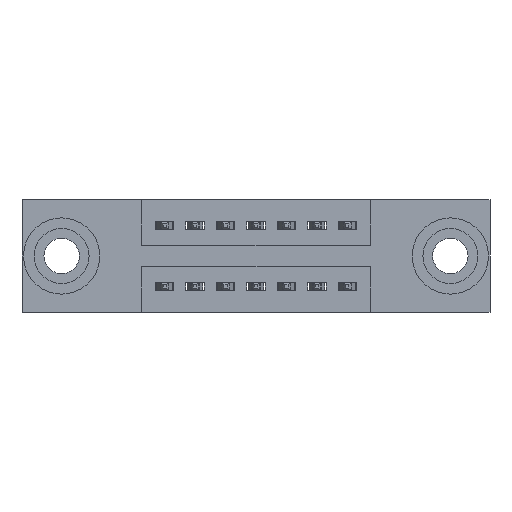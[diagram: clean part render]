
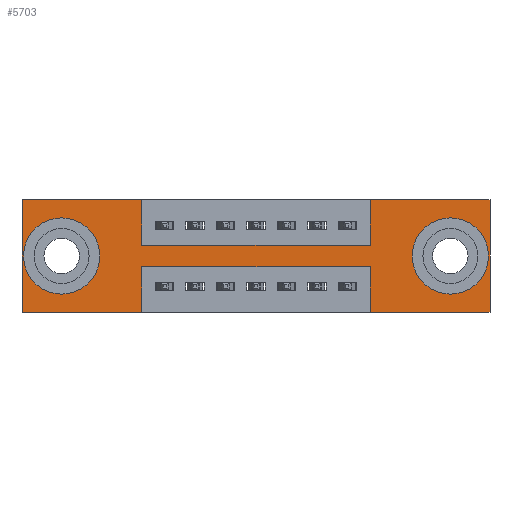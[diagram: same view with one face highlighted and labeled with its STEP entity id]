
A CAD part, front view. The second image highlights one B-rep face of the part: STEP entity #5703.
In plain terms, the highlighted planar face has unit normal (0, -1, 0).
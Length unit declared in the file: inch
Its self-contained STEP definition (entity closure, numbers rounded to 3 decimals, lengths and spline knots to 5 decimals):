
#3 = CARTESIAN_POINT ( 'NONE',  ( 0., 0., 0. ) ) ;
#21 = CARTESIAN_POINT ( 'NONE',  ( 1.405, 0., -0.185 ) ) ;
#59 = DIRECTION ( 'NONE',  ( 0., 0., -1. ) ) ;
#138 = LINE ( 'NONE', #5798, #3147 ) ;
#299 = EDGE_CURVE ( 'NONE', #4560, #1194, #5569, .T. ) ;
#536 = VECTOR ( 'NONE', #2727, 39.37008 ) ;
#591 = VECTOR ( 'NONE', #1917, 39.37008 ) ;
#703 = ORIENTED_EDGE ( 'NONE', *, *, #299, .F. ) ;
#714 = AXIS2_PLACEMENT_3D ( 'NONE', #5521, #6251, #9649 ) ;
#724 = VERTEX_POINT ( 'NONE', #5228 ) ;
#818 = EDGE_CURVE ( 'NONE', #1857, #6247, #9412, .T. ) ;
#873 = EDGE_CURVE ( 'NONE', #10096, #724, #7395, .T. ) ;
#959 = CARTESIAN_POINT ( 'NONE',  ( 0., 0., 0. ) ) ;
#982 = VERTEX_POINT ( 'NONE', #9617 ) ;
#1030 = LINE ( 'NONE', #1117, #3262 ) ;
#1117 = CARTESIAN_POINT ( 'NONE',  ( 0.3925, 0., -0.37 ) ) ;
#1194 = VERTEX_POINT ( 'NONE', #9679 ) ;
#1255 = ORIENTED_EDGE ( 'NONE', *, *, #873, .F. ) ;
#1305 = DIRECTION ( 'NONE',  ( 0., -1., 0. ) ) ;
#1344 = DIRECTION ( 'NONE',  ( 0., 0., 1. ) ) ;
#1457 = AXIS2_PLACEMENT_3D ( 'NONE', #8016, #1305, #7161 ) ;
#1614 = DIRECTION ( 'NONE',  ( 0., 0., 1. ) ) ;
#1857 = VERTEX_POINT ( 'NONE', #4517 ) ;
#1917 = DIRECTION ( 'NONE',  ( 1., 0., 0. ) ) ;
#1962 = DIRECTION ( 'NONE',  ( -1., 0., 0. ) ) ;
#2001 = LINE ( 'NONE', #5699, #6578 ) ;
#2029 = LINE ( 'NONE', #6967, #7410 ) ;
#2060 = ORIENTED_EDGE ( 'NONE', *, *, #8408, .F. ) ;
#2261 = EDGE_LOOP ( 'NONE', ( #7675, #8091 ) ) ;
#2340 = VECTOR ( 'NONE', #7805, 39.37008 ) ;
#2434 = VERTEX_POINT ( 'NONE', #9729 ) ;
#2466 = DIRECTION ( 'NONE',  ( 1., 0., 0. ) ) ;
#2493 = CIRCLE ( 'NONE', #8941, 0.078 ) ;
#2727 = DIRECTION ( 'NONE',  ( -1., 0., 0. ) ) ;
#2781 = EDGE_CURVE ( 'NONE', #982, #7110, #4473, .T. ) ;
#2797 = VERTEX_POINT ( 'NONE', #7860 ) ;
#2852 = PLANE ( 'NONE',  #1457 ) ;
#2997 = CIRCLE ( 'NONE', #8398, 0.078 ) ;
#3083 = ORIENTED_EDGE ( 'NONE', *, *, #8130, .T. ) ;
#3131 = LINE ( 'NONE', #3548, #2340 ) ;
#3147 = VECTOR ( 'NONE', #3277, 39.37008 ) ;
#3151 = CARTESIAN_POINT ( 'NONE',  ( 0., 0., 0. ) ) ;
#3242 = LINE ( 'NONE', #959, #7708 ) ;
#3262 = VECTOR ( 'NONE', #5261, 39.37008 ) ;
#3277 = DIRECTION ( 'NONE',  ( 0., 0., -1. ) ) ;
#3548 = CARTESIAN_POINT ( 'NONE',  ( 0.3925, 0., 0. ) ) ;
#3661 = LINE ( 'NONE', #5822, #7868 ) ;
#4169 = EDGE_CURVE ( 'NONE', #6126, #982, #1030, .T. ) ;
#4178 = CARTESIAN_POINT ( 'NONE',  ( 0.3925, 0., -0.22 ) ) ;
#4186 = LINE ( 'NONE', #3, #8952 ) ;
#4226 = DIRECTION ( 'NONE',  ( 0., 1., 0. ) ) ;
#4406 = ORIENTED_EDGE ( 'NONE', *, *, #9287, .F. ) ;
#4445 = CARTESIAN_POINT ( 'NONE',  ( 1.405, 0., -0.185 ) ) ;
#4462 = FACE_BOUND ( 'NONE', #7424, .T. ) ;
#4473 = LINE ( 'NONE', #7748, #536 ) ;
#4517 = CARTESIAN_POINT ( 'NONE',  ( 0.13, 0., -0.107 ) ) ;
#4531 = CARTESIAN_POINT ( 'NONE',  ( 0.3925, 0., -0.15 ) ) ;
#4560 = VERTEX_POINT ( 'NONE', #5436 ) ;
#4584 = EDGE_CURVE ( 'NONE', #2797, #4896, #2997, .T. ) ;
#4623 = AXIS2_PLACEMENT_3D ( 'NONE', #6593, #8422, #10015 ) ;
#4896 = VERTEX_POINT ( 'NONE', #6529 ) ;
#4902 = DIRECTION ( 'NONE',  ( 1., 0., 0. ) ) ;
#4935 = ORIENTED_EDGE ( 'NONE', *, *, #4169, .F. ) ;
#5064 = CIRCLE ( 'NONE', #4623, 0.078 ) ;
#5070 = EDGE_CURVE ( 'NONE', #1194, #10310, #3242, .T. ) ;
#5228 = CARTESIAN_POINT ( 'NONE',  ( 1.1425, 0., -0.22 ) ) ;
#5261 = DIRECTION ( 'NONE',  ( 0., 0., -1. ) ) ;
#5436 = CARTESIAN_POINT ( 'NONE',  ( 1.1425, 0., -0.15 ) ) ;
#5521 = CARTESIAN_POINT ( 'NONE',  ( 0.13, 0., -0.185 ) ) ;
#5569 = LINE ( 'NONE', #7599, #6995 ) ;
#5661 = CARTESIAN_POINT ( 'NONE',  ( 1.1425, 0., -0.37 ) ) ;
#5699 = CARTESIAN_POINT ( 'NONE',  ( 0., 0., 0. ) ) ;
#5703 = ADVANCED_FACE ( 'NONE', ( #7212, #4462, #5887 ), #2852, .T. ) ;
#5794 = CARTESIAN_POINT ( 'NONE',  ( 0.3925, 0., 0. ) ) ;
#5798 = CARTESIAN_POINT ( 'NONE',  ( 1.535, 0., 0. ) ) ;
#5822 = CARTESIAN_POINT ( 'NONE',  ( 0.3925, 0., -0.22 ) ) ;
#5887 = FACE_OUTER_BOUND ( 'NONE', #9410, .T. ) ;
#5891 = EDGE_CURVE ( 'NONE', #10310, #2434, #138, .T. ) ;
#5989 = EDGE_CURVE ( 'NONE', #4896, #2797, #2493, .T. ) ;
#6102 = CARTESIAN_POINT ( 'NONE',  ( 0.13, 0., -0.263 ) ) ;
#6126 = VERTEX_POINT ( 'NONE', #4178 ) ;
#6140 = EDGE_CURVE ( 'NONE', #724, #6126, #3661, .T. ) ;
#6144 = EDGE_CURVE ( 'NONE', #7110, #10516, #4186, .T. ) ;
#6157 = CARTESIAN_POINT ( 'NONE',  ( 0., 0., -0.37 ) ) ;
#6247 = VERTEX_POINT ( 'NONE', #6102 ) ;
#6251 = DIRECTION ( 'NONE',  ( 0., 1., 0. ) ) ;
#6363 = CARTESIAN_POINT ( 'NONE',  ( 1.1425, 0., -0.37 ) ) ;
#6529 = CARTESIAN_POINT ( 'NONE',  ( 1.405, 0., -0.263 ) ) ;
#6578 = VECTOR ( 'NONE', #4902, 39.37008 ) ;
#6593 = CARTESIAN_POINT ( 'NONE',  ( 0.13, 0., -0.185 ) ) ;
#6632 = DIRECTION ( 'NONE',  ( 0., 0., 1. ) ) ;
#6664 = ORIENTED_EDGE ( 'NONE', *, *, #6144, .F. ) ;
#6742 = LINE ( 'NONE', #10386, #591 ) ;
#6839 = EDGE_CURVE ( 'NONE', #8147, #8821, #3131, .T. ) ;
#6926 = CARTESIAN_POINT ( 'NONE',  ( 1.535, 0., 0. ) ) ;
#6967 = CARTESIAN_POINT ( 'NONE',  ( 0., 0., -0.37 ) ) ;
#6995 = VECTOR ( 'NONE', #6632, 39.37008 ) ;
#6998 = DIRECTION ( 'NONE',  ( 0., 0., -1. ) ) ;
#7110 = VERTEX_POINT ( 'NONE', #6157 ) ;
#7161 = DIRECTION ( 'NONE',  ( 0., 0., -1. ) ) ;
#7212 = FACE_BOUND ( 'NONE', #2261, .T. ) ;
#7395 = LINE ( 'NONE', #6363, #10454 ) ;
#7410 = VECTOR ( 'NONE', #1962, 39.37008 ) ;
#7424 = EDGE_LOOP ( 'NONE', ( #8497, #3083 ) ) ;
#7599 = CARTESIAN_POINT ( 'NONE',  ( 1.1425, 0., 0. ) ) ;
#7675 = ORIENTED_EDGE ( 'NONE', *, *, #4584, .T. ) ;
#7685 = ORIENTED_EDGE ( 'NONE', *, *, #5070, .F. ) ;
#7708 = VECTOR ( 'NONE', #2466, 39.37008 ) ;
#7748 = CARTESIAN_POINT ( 'NONE',  ( 0., 0., -0.37 ) ) ;
#7805 = DIRECTION ( 'NONE',  ( 0., 0., -1. ) ) ;
#7860 = CARTESIAN_POINT ( 'NONE',  ( 1.405, 0., -0.107 ) ) ;
#7868 = VECTOR ( 'NONE', #10008, 39.37008 ) ;
#7902 = DIRECTION ( 'NONE',  ( 0., 1., 0. ) ) ;
#8016 = CARTESIAN_POINT ( 'NONE',  ( 0., 0., -0.37 ) ) ;
#8091 = ORIENTED_EDGE ( 'NONE', *, *, #5989, .T. ) ;
#8130 = EDGE_CURVE ( 'NONE', #6247, #1857, #5064, .T. ) ;
#8147 = VERTEX_POINT ( 'NONE', #5794 ) ;
#8343 = ORIENTED_EDGE ( 'NONE', *, *, #6140, .F. ) ;
#8398 = AXIS2_PLACEMENT_3D ( 'NONE', #4445, #7902, #6998 ) ;
#8408 = EDGE_CURVE ( 'NONE', #8821, #4560, #6742, .T. ) ;
#8410 = ORIENTED_EDGE ( 'NONE', *, *, #5891, .F. ) ;
#8422 = DIRECTION ( 'NONE',  ( 0., 1., 0. ) ) ;
#8497 = ORIENTED_EDGE ( 'NONE', *, *, #818, .T. ) ;
#8691 = ORIENTED_EDGE ( 'NONE', *, *, #10041, .F. ) ;
#8821 = VERTEX_POINT ( 'NONE', #4531 ) ;
#8831 = ORIENTED_EDGE ( 'NONE', *, *, #6839, .F. ) ;
#8941 = AXIS2_PLACEMENT_3D ( 'NONE', #21, #4226, #59 ) ;
#8952 = VECTOR ( 'NONE', #1614, 39.37008 ) ;
#9020 = ORIENTED_EDGE ( 'NONE', *, *, #2781, .F. ) ;
#9287 = EDGE_CURVE ( 'NONE', #2434, #10096, #2029, .T. ) ;
#9410 = EDGE_LOOP ( 'NONE', ( #4935, #8343, #1255, #4406, #8410, #7685, #703, #2060, #8831, #8691, #6664, #9020 ) ) ;
#9412 = CIRCLE ( 'NONE', #714, 0.078 ) ;
#9617 = CARTESIAN_POINT ( 'NONE',  ( 0.3925, 0., -0.37 ) ) ;
#9649 = DIRECTION ( 'NONE',  ( 0., 0., 1. ) ) ;
#9679 = CARTESIAN_POINT ( 'NONE',  ( 1.1425, 0., 0. ) ) ;
#9729 = CARTESIAN_POINT ( 'NONE',  ( 1.535, 0., -0.37 ) ) ;
#10008 = DIRECTION ( 'NONE',  ( -1., 0., 0. ) ) ;
#10015 = DIRECTION ( 'NONE',  ( 0., 0., 1. ) ) ;
#10041 = EDGE_CURVE ( 'NONE', #10516, #8147, #2001, .T. ) ;
#10096 = VERTEX_POINT ( 'NONE', #5661 ) ;
#10310 = VERTEX_POINT ( 'NONE', #6926 ) ;
#10386 = CARTESIAN_POINT ( 'NONE',  ( 0.3925, 0., -0.15 ) ) ;
#10454 = VECTOR ( 'NONE', #1344, 39.37008 ) ;
#10516 = VERTEX_POINT ( 'NONE', #3151 ) ;
